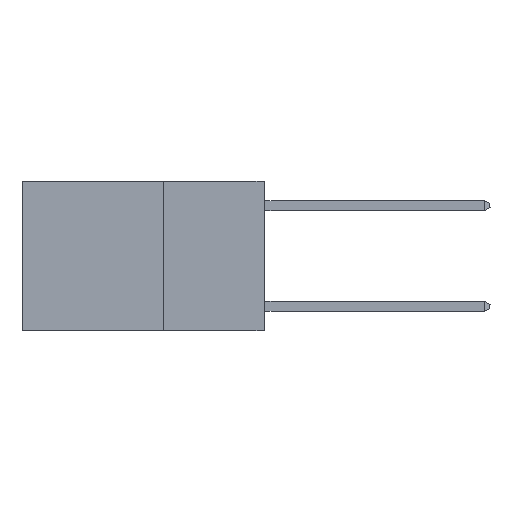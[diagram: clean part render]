
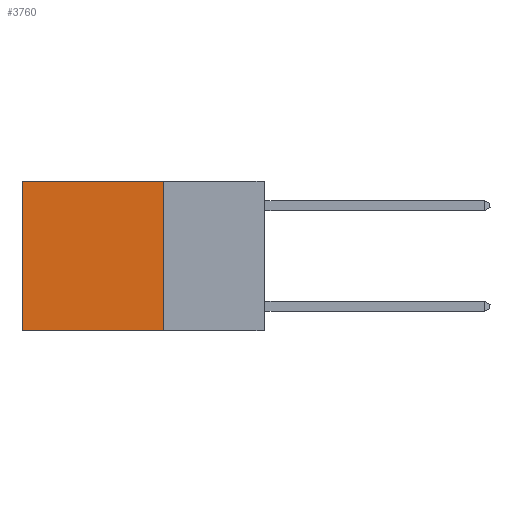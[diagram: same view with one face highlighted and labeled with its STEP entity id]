
A CAD part, left-side view. The second image highlights one B-rep face of the part: STEP entity #3760.
In plain terms, the highlighted planar face has unit normal (-1, 0, 0).
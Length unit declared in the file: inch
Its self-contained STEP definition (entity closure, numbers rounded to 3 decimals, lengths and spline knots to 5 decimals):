
#90 = VECTOR ( 'NONE', #26164, 39.37008 ) ;
#209 = CARTESIAN_POINT ( 'NONE',  ( 0.2625, 0.25, 0. ) ) ;
#362 = PLANE ( 'NONE',  #13815 ) ;
#1163 = DIRECTION ( 'NONE',  ( 0., 1., 0. ) ) ;
#3055 = ORIENTED_EDGE ( 'NONE', *, *, #27632, .F. ) ;
#3427 = LINE ( 'NONE', #5569, #90 ) ;
#3609 = CARTESIAN_POINT ( 'NONE',  ( 0.2625, 0.25, 0. ) ) ;
#3760 = ADVANCED_FACE ( 'NONE', ( #7317 ), #362, .F. ) ;
#3805 = CARTESIAN_POINT ( 'NONE',  ( 0.2625, 0.25, 0. ) ) ;
#4164 = LINE ( 'NONE', #3609, #11225 ) ;
#4958 = EDGE_LOOP ( 'NONE', ( #11391, #9038, #3055, #27642 ) ) ;
#5569 = CARTESIAN_POINT ( 'NONE',  ( 0.2625, 0.6, 0. ) ) ;
#6139 = VECTOR ( 'NONE', #18336, 39.37008 ) ;
#7317 = FACE_OUTER_BOUND ( 'NONE', #4958, .T. ) ;
#7533 = CARTESIAN_POINT ( 'NONE',  ( 0.2625, 0.25, 0. ) ) ;
#9038 = ORIENTED_EDGE ( 'NONE', *, *, #23429, .F. ) ;
#9387 = DIRECTION ( 'NONE',  ( 0., 0., -1. ) ) ;
#9669 = DIRECTION ( 'NONE',  ( 1., 0., 0. ) ) ;
#11225 = VECTOR ( 'NONE', #19075, 39.37008 ) ;
#11391 = ORIENTED_EDGE ( 'NONE', *, *, #17189, .T. ) ;
#11682 = LINE ( 'NONE', #209, #15945 ) ;
#12850 = CARTESIAN_POINT ( 'NONE',  ( 0.2625, 0.6, -0.37 ) ) ;
#13815 = AXIS2_PLACEMENT_3D ( 'NONE', #7533, #9669, #9387 ) ;
#14629 = CARTESIAN_POINT ( 'NONE',  ( 0.2625, 0.6, 0. ) ) ;
#15161 = VERTEX_POINT ( 'NONE', #12850 ) ;
#15945 = VECTOR ( 'NONE', #1163, 39.37008 ) ;
#17158 = EDGE_CURVE ( 'NONE', #17706, #20723, #11682, .T. ) ;
#17189 = EDGE_CURVE ( 'NONE', #20723, #15161, #3427, .T. ) ;
#17706 = VERTEX_POINT ( 'NONE', #3805 ) ;
#18336 = DIRECTION ( 'NONE',  ( 0., 1., 0. ) ) ;
#19075 = DIRECTION ( 'NONE',  ( 0., 0., -1. ) ) ;
#20471 = CARTESIAN_POINT ( 'NONE',  ( 0.2625, 0.25, -0.37 ) ) ;
#20723 = VERTEX_POINT ( 'NONE', #14629 ) ;
#22597 = LINE ( 'NONE', #20471, #6139 ) ;
#23429 = EDGE_CURVE ( 'NONE', #26381, #15161, #22597, .T. ) ;
#26164 = DIRECTION ( 'NONE',  ( 0., 0., -1. ) ) ;
#26381 = VERTEX_POINT ( 'NONE', #27555 ) ;
#27555 = CARTESIAN_POINT ( 'NONE',  ( 0.2625, 0.25, -0.37 ) ) ;
#27632 = EDGE_CURVE ( 'NONE', #17706, #26381, #4164, .T. ) ;
#27642 = ORIENTED_EDGE ( 'NONE', *, *, #17158, .T. ) ;
